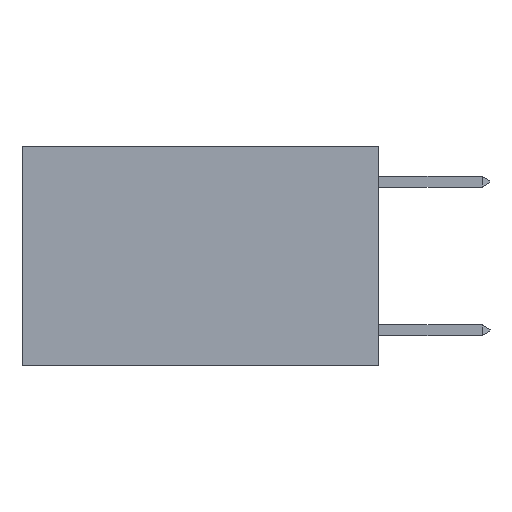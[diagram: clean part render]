
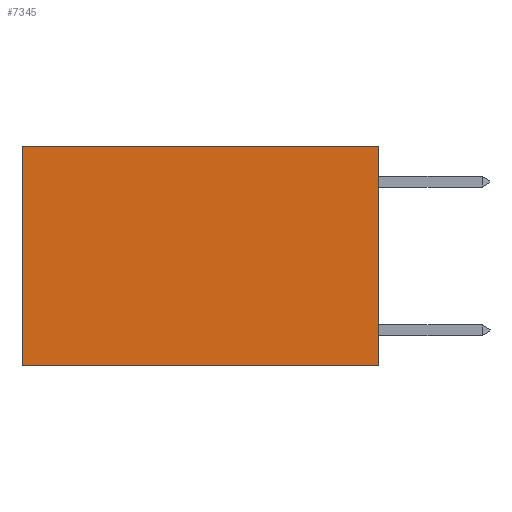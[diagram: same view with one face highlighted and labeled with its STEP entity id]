
A CAD part, left-side view. The second image highlights one B-rep face of the part: STEP entity #7345.
In plain terms, the highlighted planar face has unit normal (-1, 0, 0).
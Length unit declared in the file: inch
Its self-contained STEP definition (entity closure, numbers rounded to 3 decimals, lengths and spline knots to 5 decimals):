
#610 = VERTEX_POINT ( 'NONE', #22802 ) ;
#619 = EDGE_CURVE ( 'NONE', #610, #19656, #1151, .T. ) ;
#899 = DIRECTION ( 'NONE',  ( 0., 0., -1. ) ) ;
#923 = CARTESIAN_POINT ( 'NONE',  ( 0.2625, 0.6, -0.37 ) ) ;
#1151 = LINE ( 'NONE', #21130, #1308 ) ;
#1308 = VECTOR ( 'NONE', #3747, 39.37008 ) ;
#1782 = ORIENTED_EDGE ( 'NONE', *, *, #619, .F. ) ;
#2275 = AXIS2_PLACEMENT_3D ( 'NONE', #19151, #19127, #19120 ) ;
#3258 = VECTOR ( 'NONE', #899, 39.37008 ) ;
#3481 = LINE ( 'NONE', #6707, #3258 ) ;
#3747 = DIRECTION ( 'NONE',  ( 0., 1., 0. ) ) ;
#3867 = VECTOR ( 'NONE', #20358, 39.37008 ) ;
#3893 = LINE ( 'NONE', #14821, #3867 ) ;
#4740 = ORIENTED_EDGE ( 'NONE', *, *, #4810, .T. ) ;
#4810 = EDGE_CURVE ( 'NONE', #20612, #16223, #16170, .T. ) ;
#6707 = CARTESIAN_POINT ( 'NONE',  ( 0.2625, 0., 0. ) ) ;
#7345 = ADVANCED_FACE ( 'NONE', ( #10705 ), #19428, .F. ) ;
#9584 = CARTESIAN_POINT ( 'NONE',  ( 0.2625, 0., 0. ) ) ;
#9668 = CARTESIAN_POINT ( 'NONE',  ( 0.2625, 0.6, 0. ) ) ;
#9916 = ORIENTED_EDGE ( 'NONE', *, *, #10579, .T. ) ;
#10579 = EDGE_CURVE ( 'NONE', #16223, #19656, #3893, .T. ) ;
#10705 = FACE_OUTER_BOUND ( 'NONE', #15956, .T. ) ;
#14821 = CARTESIAN_POINT ( 'NONE',  ( 0.2625, 0.6, 0. ) ) ;
#15511 = VECTOR ( 'NONE', #22887, 39.37008 ) ;
#15956 = EDGE_LOOP ( 'NONE', ( #9916, #1782, #18410, #4740 ) ) ;
#16170 = LINE ( 'NONE', #22945, #15511 ) ;
#16223 = VERTEX_POINT ( 'NONE', #9668 ) ;
#18410 = ORIENTED_EDGE ( 'NONE', *, *, #20311, .F. ) ;
#19120 = DIRECTION ( 'NONE',  ( 0., 0., -1. ) ) ;
#19127 = DIRECTION ( 'NONE',  ( 1., 0., 0. ) ) ;
#19151 = CARTESIAN_POINT ( 'NONE',  ( 0.2625, 0., 0. ) ) ;
#19428 = PLANE ( 'NONE',  #2275 ) ;
#19656 = VERTEX_POINT ( 'NONE', #923 ) ;
#20311 = EDGE_CURVE ( 'NONE', #20612, #610, #3481, .T. ) ;
#20358 = DIRECTION ( 'NONE',  ( 0., 0., -1. ) ) ;
#20612 = VERTEX_POINT ( 'NONE', #9584 ) ;
#21130 = CARTESIAN_POINT ( 'NONE',  ( 0.2625, 0., -0.37 ) ) ;
#22802 = CARTESIAN_POINT ( 'NONE',  ( 0.2625, 0., -0.37 ) ) ;
#22887 = DIRECTION ( 'NONE',  ( 0., 1., 0. ) ) ;
#22945 = CARTESIAN_POINT ( 'NONE',  ( 0.2625, 0., 0. ) ) ;
